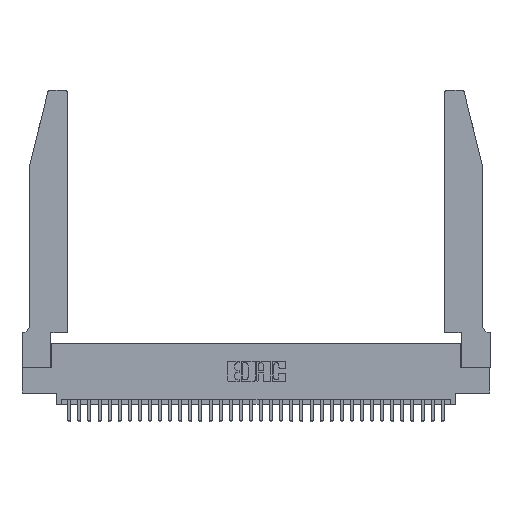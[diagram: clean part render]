
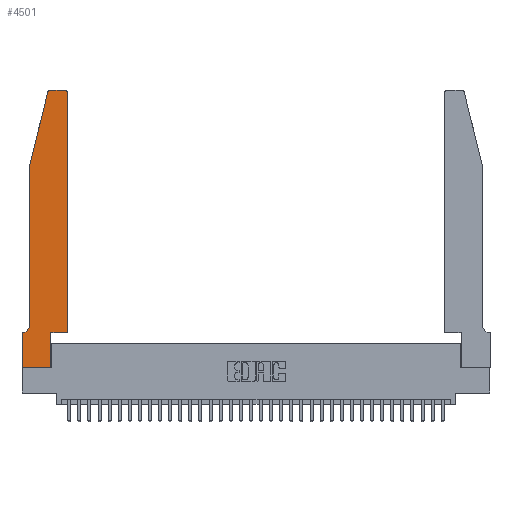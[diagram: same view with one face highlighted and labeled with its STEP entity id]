
A CAD part, top view. The second image highlights one B-rep face of the part: STEP entity #4501.
In plain terms, the highlighted planar face has unit normal (0, 0, 1).
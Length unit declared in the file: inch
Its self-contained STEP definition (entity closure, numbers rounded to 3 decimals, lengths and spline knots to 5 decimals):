
#417 = DIRECTION ( 'NONE',  ( -0.239, -0.971, 0. ) ) ;
#1006 = DIRECTION ( 'NONE',  ( 0., -1., 0. ) ) ;
#1148 = CARTESIAN_POINT ( 'NONE',  ( 0.4505, 0.35, 0.37 ) ) ;
#1183 = ORIENTED_EDGE ( 'NONE', *, *, #34458, .T. ) ;
#1205 = EDGE_CURVE ( 'NONE', #4476, #24166, #15851, .T. ) ;
#1228 = VECTOR ( 'NONE', #10352, 39.37008 ) ;
#1336 = DIRECTION ( 'NONE',  ( 0., 0., 1. ) ) ;
#1423 = EDGE_LOOP ( 'NONE', ( #1183, #14998, #2521, #20875, #11366, #5807, #26773, #21241, #6226, #29701, #24707, #26554 ) ) ;
#2050 = VERTEX_POINT ( 'NONE', #6295 ) ;
#2521 = ORIENTED_EDGE ( 'NONE', *, *, #2601, .T. ) ;
#2601 = EDGE_CURVE ( 'NONE', #22096, #16080, #31015, .T. ) ;
#2787 = CARTESIAN_POINT ( 'NONE',  ( 0.2865, 0., 0.37 ) ) ;
#3949 = EDGE_CURVE ( 'NONE', #9986, #29809, #5803, .T. ) ;
#4476 = VERTEX_POINT ( 'NONE', #8550 ) ;
#4501 = ADVANCED_FACE ( 'NONE', ( #9643 ), #22344, .T. ) ;
#4687 = EDGE_CURVE ( 'NONE', #14265, #12209, #11769, .T. ) ;
#4787 = CARTESIAN_POINT ( 'NONE',  ( 0.0755, 2., 0.37 ) ) ;
#4816 = CARTESIAN_POINT ( 'NONE',  ( 0.4505, 0.35, 0.37 ) ) ;
#5057 = DIRECTION ( 'NONE',  ( 0., 0., -1. ) ) ;
#5803 = CIRCLE ( 'NONE', #9320, 0.03 ) ;
#5807 = ORIENTED_EDGE ( 'NONE', *, *, #7441, .T. ) ;
#5904 = CARTESIAN_POINT ( 'NONE',  ( 0., 0.35, 0.37 ) ) ;
#6082 = CARTESIAN_POINT ( 'NONE',  ( 0.0055, 0.35, 0.37 ) ) ;
#6226 = ORIENTED_EDGE ( 'NONE', *, *, #4687, .T. ) ;
#6295 = CARTESIAN_POINT ( 'NONE',  ( 0.284, 2.75, 0.37 ) ) ;
#6526 = DIRECTION ( 'NONE',  ( 0., 0., 1. ) ) ;
#6739 = EDGE_CURVE ( 'NONE', #2050, #22096, #26700, .T. ) ;
#7441 = EDGE_CURVE ( 'NONE', #24166, #16939, #27072, .T. ) ;
#8550 = CARTESIAN_POINT ( 'NONE',  ( 0.0755, 0.42, 0.37 ) ) ;
#9320 = AXIS2_PLACEMENT_3D ( 'NONE', #22977, #6526, #25707 ) ;
#9531 = CARTESIAN_POINT ( 'NONE',  ( 0.0755, 0.35, 0.37 ) ) ;
#9643 = FACE_OUTER_BOUND ( 'NONE', #1423, .T. ) ;
#9986 = VERTEX_POINT ( 'NONE', #26601 ) ;
#10352 = DIRECTION ( 'NONE',  ( -1., 0., 0. ) ) ;
#10456 = VECTOR ( 'NONE', #23974, 39.37008 ) ;
#11021 = VECTOR ( 'NONE', #417, 39.37008 ) ;
#11366 = ORIENTED_EDGE ( 'NONE', *, *, #1205, .T. ) ;
#11423 = DIRECTION ( 'NONE',  ( 1., 0., 0. ) ) ;
#11769 = LINE ( 'NONE', #14789, #26347 ) ;
#11785 = VERTEX_POINT ( 'NONE', #4816 ) ;
#12209 = VERTEX_POINT ( 'NONE', #34206 ) ;
#12248 = DIRECTION ( 'NONE',  ( 0., 1., 0. ) ) ;
#12356 = LINE ( 'NONE', #14777, #26076 ) ;
#14265 = VERTEX_POINT ( 'NONE', #2787 ) ;
#14777 = CARTESIAN_POINT ( 'NONE',  ( 0., 0., 0.37 ) ) ;
#14789 = CARTESIAN_POINT ( 'NONE',  ( 0.2865, 0.35, 0.37 ) ) ;
#14808 = CARTESIAN_POINT ( 'NONE',  ( 0., 0., 0.37 ) ) ;
#14906 = CARTESIAN_POINT ( 'NONE',  ( 0.25487, 2.72718, 0.37 ) ) ;
#14998 = ORIENTED_EDGE ( 'NONE', *, *, #6739, .T. ) ;
#15139 = EDGE_CURVE ( 'NONE', #11785, #9986, #35046, .T. ) ;
#15851 = CIRCLE ( 'NONE', #28246, 0.07 ) ;
#16080 = VERTEX_POINT ( 'NONE', #21323 ) ;
#16793 = LINE ( 'NONE', #34715, #1228 ) ;
#16900 = LINE ( 'NONE', #4787, #10456 ) ;
#16939 = VERTEX_POINT ( 'NONE', #19577 ) ;
#17219 = AXIS2_PLACEMENT_3D ( 'NONE', #17883, #1336, #20622 ) ;
#17527 = VECTOR ( 'NONE', #29482, 39.37008 ) ;
#17582 = DIRECTION ( 'NONE',  ( 1., 0., 0. ) ) ;
#17883 = CARTESIAN_POINT ( 'NONE',  ( 0.284, 2.72, 0.37 ) ) ;
#18120 = LINE ( 'NONE', #14808, #31649 ) ;
#18393 = LINE ( 'NONE', #24090, #17527 ) ;
#19010 = VECTOR ( 'NONE', #31325, 39.37008 ) ;
#19577 = CARTESIAN_POINT ( 'NONE',  ( 0., 0.35, 0.37 ) ) ;
#20242 = EDGE_CURVE ( 'NONE', #16939, #27432, #12356, .T. ) ;
#20510 = EDGE_CURVE ( 'NONE', #12209, #11785, #18393, .T. ) ;
#20622 = DIRECTION ( 'NONE',  ( 1., 0., 0. ) ) ;
#20875 = ORIENTED_EDGE ( 'NONE', *, *, #23835, .T. ) ;
#21241 = ORIENTED_EDGE ( 'NONE', *, *, #34177, .T. ) ;
#21323 = CARTESIAN_POINT ( 'NONE',  ( 0.0755, 2., 0.37 ) ) ;
#22096 = VERTEX_POINT ( 'NONE', #14906 ) ;
#22344 = PLANE ( 'NONE',  #32372 ) ;
#22977 = CARTESIAN_POINT ( 'NONE',  ( 0.4205, 2.72, 0.37 ) ) ;
#23835 = EDGE_CURVE ( 'NONE', #16080, #4476, #16900, .T. ) ;
#23974 = DIRECTION ( 'NONE',  ( 0., -1., 0. ) ) ;
#24090 = CARTESIAN_POINT ( 'NONE',  ( 0.4505, 0.35, 0.37 ) ) ;
#24166 = VERTEX_POINT ( 'NONE', #6082 ) ;
#24707 = ORIENTED_EDGE ( 'NONE', *, *, #15139, .T. ) ;
#25063 = DIRECTION ( 'NONE',  ( -1., 0., 0. ) ) ;
#25229 = CARTESIAN_POINT ( 'NONE',  ( 0.0055, 0.42, 0.37 ) ) ;
#25707 = DIRECTION ( 'NONE',  ( 1., 0., 0. ) ) ;
#26076 = VECTOR ( 'NONE', #1006, 39.37008 ) ;
#26347 = VECTOR ( 'NONE', #33770, 39.37008 ) ;
#26554 = ORIENTED_EDGE ( 'NONE', *, *, #3949, .T. ) ;
#26601 = CARTESIAN_POINT ( 'NONE',  ( 0.4505, 2.72, 0.37 ) ) ;
#26700 = CIRCLE ( 'NONE', #17219, 0.03 ) ;
#26773 = ORIENTED_EDGE ( 'NONE', *, *, #20242, .T. ) ;
#27072 = LINE ( 'NONE', #9531, #19010 ) ;
#27432 = VERTEX_POINT ( 'NONE', #27445 ) ;
#27445 = CARTESIAN_POINT ( 'NONE',  ( 0., 0., 0.37 ) ) ;
#27784 = DIRECTION ( 'NONE',  ( 0., 0., 1. ) ) ;
#28246 = AXIS2_PLACEMENT_3D ( 'NONE', #25229, #5057, #25063 ) ;
#29482 = DIRECTION ( 'NONE',  ( 1., 0., 0. ) ) ;
#29701 = ORIENTED_EDGE ( 'NONE', *, *, #20510, .T. ) ;
#29809 = VERTEX_POINT ( 'NONE', #31920 ) ;
#31015 = LINE ( 'NONE', #33179, #11021 ) ;
#31325 = DIRECTION ( 'NONE',  ( -1., 0., 0. ) ) ;
#31649 = VECTOR ( 'NONE', #17582, 39.37008 ) ;
#31920 = CARTESIAN_POINT ( 'NONE',  ( 0.4205, 2.75, 0.37 ) ) ;
#32372 = AXIS2_PLACEMENT_3D ( 'NONE', #5904, #27784, #11423 ) ;
#33179 = CARTESIAN_POINT ( 'NONE',  ( 0.0755, 2., 0.37 ) ) ;
#33770 = DIRECTION ( 'NONE',  ( 0., 1., 0. ) ) ;
#34177 = EDGE_CURVE ( 'NONE', #27432, #14265, #18120, .T. ) ;
#34206 = CARTESIAN_POINT ( 'NONE',  ( 0.2865, 0.35, 0.37 ) ) ;
#34218 = VECTOR ( 'NONE', #12248, 39.37008 ) ;
#34458 = EDGE_CURVE ( 'NONE', #29809, #2050, #16793, .T. ) ;
#34715 = CARTESIAN_POINT ( 'NONE',  ( 0.2605, 2.75, 0.37 ) ) ;
#35046 = LINE ( 'NONE', #1148, #34218 ) ;
